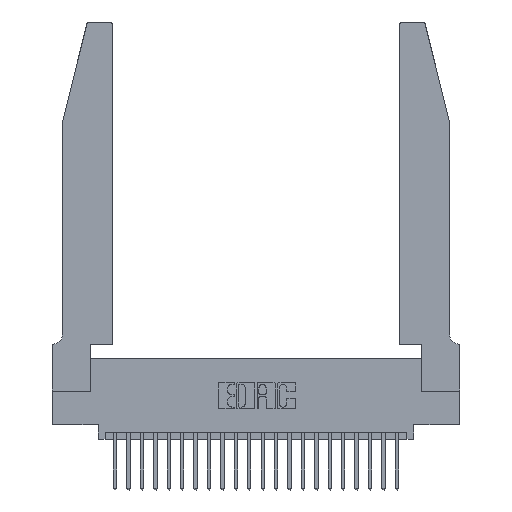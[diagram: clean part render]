
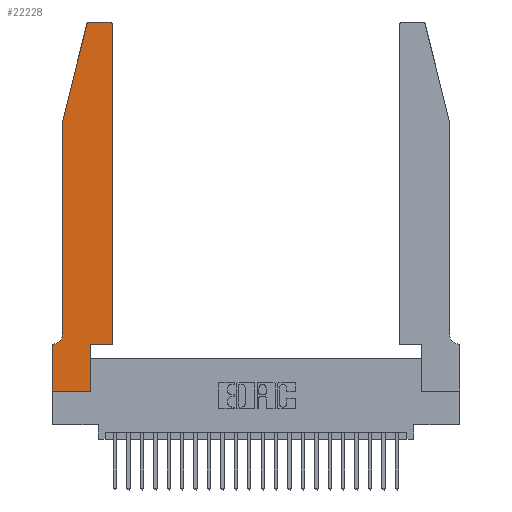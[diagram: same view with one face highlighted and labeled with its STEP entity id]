
A CAD part, top view. The second image highlights one B-rep face of the part: STEP entity #22228.
In plain terms, the highlighted planar face has unit normal (0, 0, 1).
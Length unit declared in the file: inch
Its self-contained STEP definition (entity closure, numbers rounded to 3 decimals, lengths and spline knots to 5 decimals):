
#549 = EDGE_CURVE ( 'NONE', #22989, #1000, #9516, .T. ) ;
#947 = CARTESIAN_POINT ( 'NONE',  ( 0.284, 2.75, 0.37 ) ) ;
#1000 = VERTEX_POINT ( 'NONE', #947 ) ;
#1049 = FACE_OUTER_BOUND ( 'NONE', #7606, .T. ) ;
#1449 = DIRECTION ( 'NONE',  ( 0., 0., -1. ) ) ;
#1520 = ORIENTED_EDGE ( 'NONE', *, *, #21143, .T. ) ;
#1760 = ORIENTED_EDGE ( 'NONE', *, *, #6008, .T. ) ;
#2013 = VECTOR ( 'NONE', #17630, 39.37008 ) ;
#2072 = VECTOR ( 'NONE', #21252, 39.37008 ) ;
#2422 = VECTOR ( 'NONE', #6339, 39.37008 ) ;
#2529 = EDGE_CURVE ( 'NONE', #6503, #9656, #17794, .T. ) ;
#3008 = CARTESIAN_POINT ( 'NONE',  ( 0.2605, 2.75, 0.37 ) ) ;
#4101 = CIRCLE ( 'NONE', #18188, 0.03 ) ;
#4182 = ORIENTED_EDGE ( 'NONE', *, *, #11491, .T. ) ;
#4554 = ORIENTED_EDGE ( 'NONE', *, *, #8291, .T. ) ;
#4715 = VECTOR ( 'NONE', #12734, 39.37008 ) ;
#4859 = DIRECTION ( 'NONE',  ( 0., 0., 1. ) ) ;
#5317 = AXIS2_PLACEMENT_3D ( 'NONE', #18336, #6842, #20226 ) ;
#5675 = CARTESIAN_POINT ( 'NONE',  ( 0.0755, 2., 0.37 ) ) ;
#6008 = EDGE_CURVE ( 'NONE', #9656, #22989, #4101, .T. ) ;
#6015 = CARTESIAN_POINT ( 'NONE',  ( 0., 0., 0.37 ) ) ;
#6214 = LINE ( 'NONE', #8302, #24778 ) ;
#6311 = ORIENTED_EDGE ( 'NONE', *, *, #19793, .T. ) ;
#6339 = DIRECTION ( 'NONE',  ( 0., 1., 0. ) ) ;
#6441 = DIRECTION ( 'NONE',  ( 0., 1., 0. ) ) ;
#6503 = VERTEX_POINT ( 'NONE', #23606 ) ;
#6842 = DIRECTION ( 'NONE',  ( 0., 0., 1. ) ) ;
#6909 = CARTESIAN_POINT ( 'NONE',  ( 0.0755, 2., 0.37 ) ) ;
#7195 = LINE ( 'NONE', #6015, #2013 ) ;
#7339 = CARTESIAN_POINT ( 'NONE',  ( 0.0055, 0.35, 0.37 ) ) ;
#7606 = EDGE_LOOP ( 'NONE', ( #17462, #22041, #20441, #6311, #21668, #18419, #4554, #1520, #10048, #4182, #14204, #1760 ) ) ;
#8291 = EDGE_CURVE ( 'NONE', #21482, #15406, #13577, .T. ) ;
#8302 = CARTESIAN_POINT ( 'NONE',  ( 0.0755, 0.35, 0.37 ) ) ;
#8323 = CARTESIAN_POINT ( 'NONE',  ( 0.2865, 0.35, 0.37 ) ) ;
#9179 = VECTOR ( 'NONE', #6441, 39.37008 ) ;
#9516 = LINE ( 'NONE', #3008, #24720 ) ;
#9656 = VERTEX_POINT ( 'NONE', #18052 ) ;
#9844 = VECTOR ( 'NONE', #15285, 39.37008 ) ;
#9939 = AXIS2_PLACEMENT_3D ( 'NONE', #16404, #4859, #18326 ) ;
#10048 = ORIENTED_EDGE ( 'NONE', *, *, #12956, .T. ) ;
#10278 = LINE ( 'NONE', #5675, #19808 ) ;
#10404 = VERTEX_POINT ( 'NONE', #19991 ) ;
#10432 = VERTEX_POINT ( 'NONE', #14607 ) ;
#10466 = LINE ( 'NONE', #20919, #9844 ) ;
#10644 = PLANE ( 'NONE',  #9939 ) ;
#10985 = CARTESIAN_POINT ( 'NONE',  ( 0.4205, 2.72, 0.37 ) ) ;
#11491 = EDGE_CURVE ( 'NONE', #24566, #6503, #10466, .T. ) ;
#12004 = CARTESIAN_POINT ( 'NONE',  ( 0.2865, 0.35, 0.37 ) ) ;
#12734 = DIRECTION ( 'NONE',  ( -0.239, -0.971, 0. ) ) ;
#12911 = DIRECTION ( 'NONE',  ( 1., 0., 0. ) ) ;
#12956 = EDGE_CURVE ( 'NONE', #10404, #24566, #19338, .T. ) ;
#13041 = CARTESIAN_POINT ( 'NONE',  ( 0.4205, 2.75, 0.37 ) ) ;
#13045 = CARTESIAN_POINT ( 'NONE',  ( 0.0055, 0.42, 0.37 ) ) ;
#13577 = LINE ( 'NONE', #23144, #2072 ) ;
#14030 = CARTESIAN_POINT ( 'NONE',  ( 0.4505, 0.35, 0.37 ) ) ;
#14204 = ORIENTED_EDGE ( 'NONE', *, *, #2529, .T. ) ;
#14441 = EDGE_CURVE ( 'NONE', #16310, #18216, #15593, .T. ) ;
#14607 = CARTESIAN_POINT ( 'NONE',  ( 0.0755, 0.42, 0.37 ) ) ;
#14981 = DIRECTION ( 'NONE',  ( -1., 0., 0. ) ) ;
#15285 = DIRECTION ( 'NONE',  ( 1., 0., 0. ) ) ;
#15406 = VERTEX_POINT ( 'NONE', #23215 ) ;
#15593 = LINE ( 'NONE', #6909, #4715 ) ;
#16310 = VERTEX_POINT ( 'NONE', #22517 ) ;
#16404 = CARTESIAN_POINT ( 'NONE',  ( 0., 0.35, 0.37 ) ) ;
#17462 = ORIENTED_EDGE ( 'NONE', *, *, #549, .T. ) ;
#17630 = DIRECTION ( 'NONE',  ( 1., 0., 0. ) ) ;
#17794 = LINE ( 'NONE', #14030, #2422 ) ;
#17904 = DIRECTION ( 'NONE',  ( -1., 0., 0. ) ) ;
#18052 = CARTESIAN_POINT ( 'NONE',  ( 0.4505, 2.72, 0.37 ) ) ;
#18188 = AXIS2_PLACEMENT_3D ( 'NONE', #10985, #24309, #12911 ) ;
#18216 = VERTEX_POINT ( 'NONE', #22713 ) ;
#18326 = DIRECTION ( 'NONE',  ( 1., 0., 0. ) ) ;
#18336 = CARTESIAN_POINT ( 'NONE',  ( 0.284, 2.72, 0.37 ) ) ;
#18419 = ORIENTED_EDGE ( 'NONE', *, *, #21812, .T. ) ;
#18437 = EDGE_CURVE ( 'NONE', #1000, #16310, #19285, .T. ) ;
#19285 = CIRCLE ( 'NONE', #5317, 0.03 ) ;
#19338 = LINE ( 'NONE', #8323, #9179 ) ;
#19793 = EDGE_CURVE ( 'NONE', #18216, #10432, #10278, .T. ) ;
#19808 = VECTOR ( 'NONE', #21012, 39.37008 ) ;
#19991 = CARTESIAN_POINT ( 'NONE',  ( 0.2865, 0., 0.37 ) ) ;
#20226 = DIRECTION ( 'NONE',  ( 1., 0., 0. ) ) ;
#20319 = AXIS2_PLACEMENT_3D ( 'NONE', #13045, #1449, #14981 ) ;
#20441 = ORIENTED_EDGE ( 'NONE', *, *, #14441, .T. ) ;
#20883 = VERTEX_POINT ( 'NONE', #7339 ) ;
#20919 = CARTESIAN_POINT ( 'NONE',  ( 0.4505, 0.35, 0.37 ) ) ;
#21012 = DIRECTION ( 'NONE',  ( 0., -1., 0. ) ) ;
#21143 = EDGE_CURVE ( 'NONE', #15406, #10404, #7195, .T. ) ;
#21252 = DIRECTION ( 'NONE',  ( 0., -1., 0. ) ) ;
#21434 = EDGE_CURVE ( 'NONE', #10432, #20883, #23600, .T. ) ;
#21482 = VERTEX_POINT ( 'NONE', #22580 ) ;
#21668 = ORIENTED_EDGE ( 'NONE', *, *, #21434, .T. ) ;
#21812 = EDGE_CURVE ( 'NONE', #20883, #21482, #6214, .T. ) ;
#22041 = ORIENTED_EDGE ( 'NONE', *, *, #18437, .T. ) ;
#22228 = ADVANCED_FACE ( 'NONE', ( #1049 ), #10644, .T. ) ;
#22517 = CARTESIAN_POINT ( 'NONE',  ( 0.25487, 2.72718, 0.37 ) ) ;
#22580 = CARTESIAN_POINT ( 'NONE',  ( 0., 0.35, 0.37 ) ) ;
#22713 = CARTESIAN_POINT ( 'NONE',  ( 0.0755, 2., 0.37 ) ) ;
#22989 = VERTEX_POINT ( 'NONE', #13041 ) ;
#23144 = CARTESIAN_POINT ( 'NONE',  ( 0., 0., 0.37 ) ) ;
#23215 = CARTESIAN_POINT ( 'NONE',  ( 0., 0., 0.37 ) ) ;
#23576 = DIRECTION ( 'NONE',  ( -1., 0., 0. ) ) ;
#23600 = CIRCLE ( 'NONE', #20319, 0.07 ) ;
#23606 = CARTESIAN_POINT ( 'NONE',  ( 0.4505, 0.35, 0.37 ) ) ;
#24309 = DIRECTION ( 'NONE',  ( 0., 0., 1. ) ) ;
#24566 = VERTEX_POINT ( 'NONE', #12004 ) ;
#24720 = VECTOR ( 'NONE', #17904, 39.37008 ) ;
#24778 = VECTOR ( 'NONE', #23576, 39.37008 ) ;
